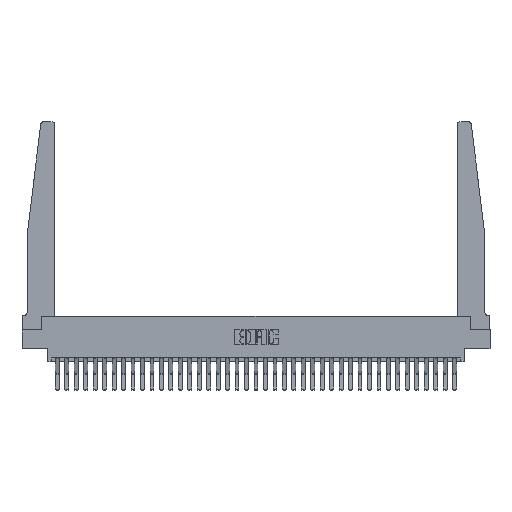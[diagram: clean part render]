
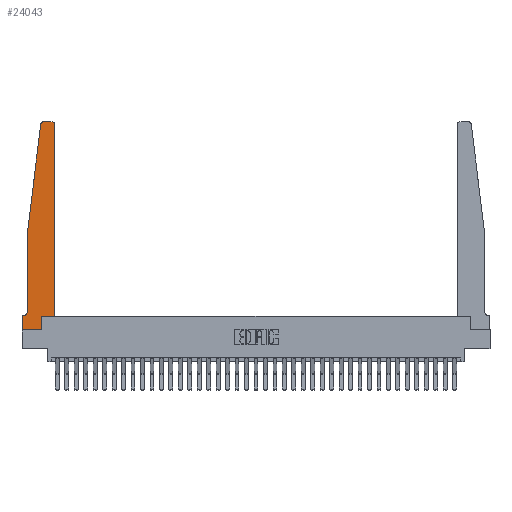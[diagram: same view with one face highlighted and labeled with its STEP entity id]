
A CAD part, top view. The second image highlights one B-rep face of the part: STEP entity #24043.
In plain terms, the highlighted planar face has unit normal (0, 0, 1).
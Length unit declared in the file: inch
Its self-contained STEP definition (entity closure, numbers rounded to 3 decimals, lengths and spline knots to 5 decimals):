
#371 = VECTOR ( 'NONE', #21238, 39.37008 ) ;
#408 = CIRCLE ( 'NONE', #4188, 0.03 ) ;
#409 = VERTEX_POINT ( 'NONE', #5841 ) ;
#677 = EDGE_CURVE ( 'NONE', #2539, #8400, #2584, .T. ) ;
#710 = VERTEX_POINT ( 'NONE', #30955 ) ;
#1504 = CARTESIAN_POINT ( 'NONE',  ( 0.425, 0.18, 0.37 ) ) ;
#2188 = DIRECTION ( 'NONE',  ( 1., 0., 0. ) ) ;
#2263 = CARTESIAN_POINT ( 'NONE',  ( 0.425, 0.18, 0.37 ) ) ;
#2539 = VERTEX_POINT ( 'NONE', #16886 ) ;
#2584 = LINE ( 'NONE', #2263, #20907 ) ;
#2931 = CARTESIAN_POINT ( 'NONE',  ( 0.425, 2.72, 0.37 ) ) ;
#2933 = EDGE_CURVE ( 'NONE', #8400, #15481, #408, .T. ) ;
#3271 = VECTOR ( 'NONE', #25296, 39.37008 ) ;
#3832 = CARTESIAN_POINT ( 'NONE',  ( 0.395, 2.72, 0.37 ) ) ;
#4034 = ORIENTED_EDGE ( 'NONE', *, *, #26208, .T. ) ;
#4114 = LINE ( 'NONE', #21372, #27124 ) ;
#4142 = CARTESIAN_POINT ( 'NONE',  ( 0.27653, 2.75, 0.37 ) ) ;
#4188 = AXIS2_PLACEMENT_3D ( 'NONE', #3832, #29860, #11106 ) ;
#4537 = CARTESIAN_POINT ( 'NONE',  ( 0.015, 0.2375, 0.37 ) ) ;
#4715 = CARTESIAN_POINT ( 'NONE',  ( 0., 0., 0.37 ) ) ;
#4886 = DIRECTION ( 'NONE',  ( 0., 0., 1. ) ) ;
#5105 = LINE ( 'NONE', #13556, #25997 ) ;
#5841 = CARTESIAN_POINT ( 'NONE',  ( 0., 0.1875, 0.37 ) ) ;
#7373 = LINE ( 'NONE', #9401, #3271 ) ;
#7404 = ORIENTED_EDGE ( 'NONE', *, *, #10926, .T. ) ;
#7619 = CARTESIAN_POINT ( 'NONE',  ( 0.065, 0.2375, 0.37 ) ) ;
#7794 = ORIENTED_EDGE ( 'NONE', *, *, #20817, .T. ) ;
#8087 = AXIS2_PLACEMENT_3D ( 'NONE', #9447, #4886, #12650 ) ;
#8400 = VERTEX_POINT ( 'NONE', #2931 ) ;
#9401 = CARTESIAN_POINT ( 'NONE',  ( 0.065, 1.25, 0.37 ) ) ;
#9424 = CARTESIAN_POINT ( 'NONE',  ( 0.015, 0.1875, 0.37 ) ) ;
#9447 = CARTESIAN_POINT ( 'NONE',  ( 0., 0.1875, 0.37 ) ) ;
#9454 = DIRECTION ( 'NONE',  ( 0., -1., 0. ) ) ;
#9587 = VECTOR ( 'NONE', #2188, 39.37008 ) ;
#9639 = ORIENTED_EDGE ( 'NONE', *, *, #677, .T. ) ;
#10187 = DIRECTION ( 'NONE',  ( 0., 1., 0. ) ) ;
#10275 = ORIENTED_EDGE ( 'NONE', *, *, #19758, .T. ) ;
#10926 = EDGE_CURVE ( 'NONE', #23588, #28689, #20728, .T. ) ;
#11006 = ORIENTED_EDGE ( 'NONE', *, *, #28439, .T. ) ;
#11106 = DIRECTION ( 'NONE',  ( 1., 0., 0. ) ) ;
#11215 = AXIS2_PLACEMENT_3D ( 'NONE', #4537, #17214, #14847 ) ;
#11664 = CARTESIAN_POINT ( 'NONE',  ( 0.065, 0.1875, 0.37 ) ) ;
#11725 = CARTESIAN_POINT ( 'NONE',  ( 0.27653, 2.72, 0.37 ) ) ;
#12650 = DIRECTION ( 'NONE',  ( 1., 0., 0. ) ) ;
#13556 = CARTESIAN_POINT ( 'NONE',  ( 0.25, 2.75, 0.37 ) ) ;
#13623 = EDGE_CURVE ( 'NONE', #14979, #710, #20425, .T. ) ;
#13870 = LINE ( 'NONE', #11664, #21701 ) ;
#13941 = DIRECTION ( 'NONE',  ( 0., 0., 1. ) ) ;
#14183 = LINE ( 'NONE', #1504, #30844 ) ;
#14416 = VERTEX_POINT ( 'NONE', #7619 ) ;
#14694 = FACE_OUTER_BOUND ( 'NONE', #20971, .T. ) ;
#14847 = DIRECTION ( 'NONE',  ( -1., 0., 0. ) ) ;
#14979 = VERTEX_POINT ( 'NONE', #29538 ) ;
#15481 = VERTEX_POINT ( 'NONE', #28828 ) ;
#15546 = CARTESIAN_POINT ( 'NONE',  ( 0.2605, 0.18, 0.37 ) ) ;
#15823 = CARTESIAN_POINT ( 'NONE',  ( 0.065, 1.25, 0.37 ) ) ;
#15977 = EDGE_CURVE ( 'NONE', #409, #14979, #28050, .T. ) ;
#16398 = DIRECTION ( 'NONE',  ( -1., 0., 0. ) ) ;
#16886 = CARTESIAN_POINT ( 'NONE',  ( 0.425, 0.18, 0.37 ) ) ;
#17214 = DIRECTION ( 'NONE',  ( 0., 0., -1. ) ) ;
#18051 = ORIENTED_EDGE ( 'NONE', *, *, #24415, .T. ) ;
#18278 = DIRECTION ( 'NONE',  ( -1., 0., 0. ) ) ;
#18415 = ORIENTED_EDGE ( 'NONE', *, *, #15977, .T. ) ;
#19758 = EDGE_CURVE ( 'NONE', #710, #21197, #4114, .T. ) ;
#19936 = PLANE ( 'NONE',  #8087 ) ;
#20425 = LINE ( 'NONE', #4715, #9587 ) ;
#20622 = CIRCLE ( 'NONE', #31403, 0.03 ) ;
#20728 = LINE ( 'NONE', #15823, #371 ) ;
#20817 = EDGE_CURVE ( 'NONE', #15481, #25300, #5105, .T. ) ;
#20907 = VECTOR ( 'NONE', #10187, 39.37008 ) ;
#20971 = EDGE_LOOP ( 'NONE', ( #7794, #11006, #7404, #18051, #25702, #27566, #18415, #30208, #10275, #4034, #9639, #22615 ) ) ;
#21197 = VERTEX_POINT ( 'NONE', #15546 ) ;
#21238 = DIRECTION ( 'NONE',  ( -0.122, -0.992, 0. ) ) ;
#21372 = CARTESIAN_POINT ( 'NONE',  ( 0.2605, 0.18, 0.37 ) ) ;
#21559 = EDGE_CURVE ( 'NONE', #14416, #31259, #25784, .T. ) ;
#21701 = VECTOR ( 'NONE', #16398, 39.37008 ) ;
#21704 = CARTESIAN_POINT ( 'NONE',  ( 0.24675, 2.72367, 0.37 ) ) ;
#22041 = DIRECTION ( 'NONE',  ( 1., 0., 0. ) ) ;
#22615 = ORIENTED_EDGE ( 'NONE', *, *, #2933, .T. ) ;
#23356 = CARTESIAN_POINT ( 'NONE',  ( 0.065, 1.25, 0.37 ) ) ;
#23588 = VERTEX_POINT ( 'NONE', #21704 ) ;
#24043 = ADVANCED_FACE ( 'NONE', ( #14694 ), #19936, .T. ) ;
#24415 = EDGE_CURVE ( 'NONE', #28689, #14416, #7373, .T. ) ;
#24788 = VECTOR ( 'NONE', #9454, 39.37008 ) ;
#25296 = DIRECTION ( 'NONE',  ( 0., -1., 0. ) ) ;
#25300 = VERTEX_POINT ( 'NONE', #4142 ) ;
#25702 = ORIENTED_EDGE ( 'NONE', *, *, #21559, .T. ) ;
#25784 = CIRCLE ( 'NONE', #11215, 0.05 ) ;
#25997 = VECTOR ( 'NONE', #18278, 39.37008 ) ;
#26208 = EDGE_CURVE ( 'NONE', #21197, #2539, #14183, .T. ) ;
#27124 = VECTOR ( 'NONE', #29151, 39.37008 ) ;
#27384 = CARTESIAN_POINT ( 'NONE',  ( 0., 0., 0.37 ) ) ;
#27566 = ORIENTED_EDGE ( 'NONE', *, *, #29123, .T. ) ;
#28050 = LINE ( 'NONE', #27384, #24788 ) ;
#28439 = EDGE_CURVE ( 'NONE', #25300, #23588, #20622, .T. ) ;
#28689 = VERTEX_POINT ( 'NONE', #23356 ) ;
#28828 = CARTESIAN_POINT ( 'NONE',  ( 0.395, 2.75, 0.37 ) ) ;
#29123 = EDGE_CURVE ( 'NONE', #31259, #409, #13870, .T. ) ;
#29151 = DIRECTION ( 'NONE',  ( 0., 1., 0. ) ) ;
#29538 = CARTESIAN_POINT ( 'NONE',  ( 0., 0., 0.37 ) ) ;
#29860 = DIRECTION ( 'NONE',  ( 0., 0., 1. ) ) ;
#30208 = ORIENTED_EDGE ( 'NONE', *, *, #13623, .T. ) ;
#30844 = VECTOR ( 'NONE', #32248, 39.37008 ) ;
#30955 = CARTESIAN_POINT ( 'NONE',  ( 0.2605, 0., 0.37 ) ) ;
#31259 = VERTEX_POINT ( 'NONE', #9424 ) ;
#31403 = AXIS2_PLACEMENT_3D ( 'NONE', #11725, #13941, #22041 ) ;
#32248 = DIRECTION ( 'NONE',  ( 1., 0., 0. ) ) ;
